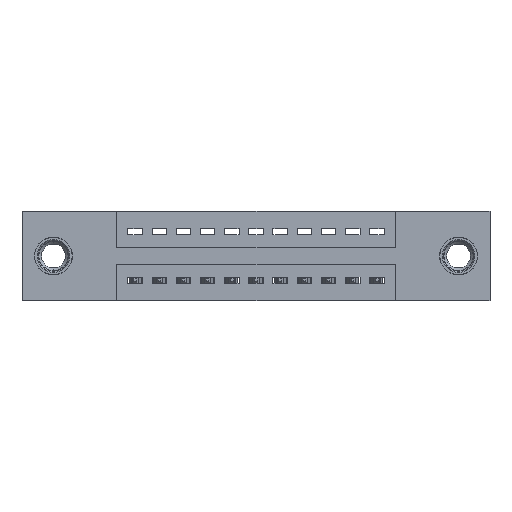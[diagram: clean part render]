
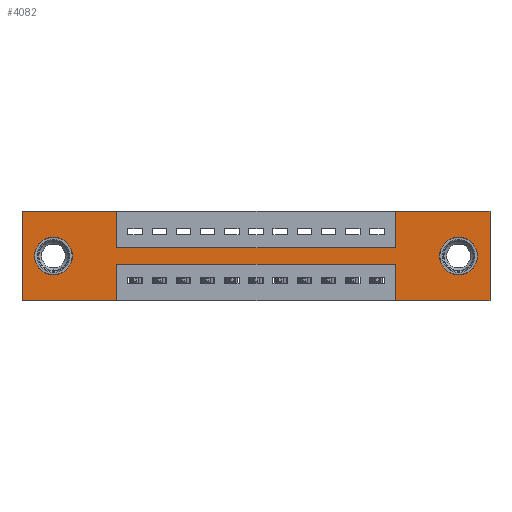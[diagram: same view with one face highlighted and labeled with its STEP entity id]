
A CAD part, front view. The second image highlights one B-rep face of the part: STEP entity #4082.
In plain terms, the highlighted planar face has unit normal (0, -1, 0).
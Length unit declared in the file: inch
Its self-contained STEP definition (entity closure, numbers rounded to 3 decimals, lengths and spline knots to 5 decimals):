
#13 = CARTESIAN_POINT ( 'NONE',  ( 0.3925, 0., -0.22 ) ) ;
#26 = CARTESIAN_POINT ( 'NONE',  ( 0.3925, 0., 0. ) ) ;
#40 = EDGE_CURVE ( 'NONE', #13042, #10069, #11287, .T. ) ;
#280 = ORIENTED_EDGE ( 'NONE', *, *, #3302, .F. ) ;
#438 = DIRECTION ( 'NONE',  ( 0., 0., 1. ) ) ;
#495 = CARTESIAN_POINT ( 'NONE',  ( 0.13, 0., -0.185 ) ) ;
#990 = VERTEX_POINT ( 'NONE', #8089 ) ;
#1061 = CARTESIAN_POINT ( 'NONE',  ( 1.805, 0., -0.185 ) ) ;
#1088 = LINE ( 'NONE', #1348, #12640 ) ;
#1348 = CARTESIAN_POINT ( 'NONE',  ( 0., 0., 0. ) ) ;
#1362 = LINE ( 'NONE', #9178, #10971 ) ;
#1451 = CARTESIAN_POINT ( 'NONE',  ( 0., 0., 0. ) ) ;
#1466 = LINE ( 'NONE', #7361, #10220 ) ;
#1479 = CARTESIAN_POINT ( 'NONE',  ( 0.3925, 0., -0.22 ) ) ;
#1532 = VERTEX_POINT ( 'NONE', #8719 ) ;
#1937 = LINE ( 'NONE', #2942, #3266 ) ;
#1959 = CARTESIAN_POINT ( 'NONE',  ( 1.5425, 0., -0.37 ) ) ;
#2083 = CARTESIAN_POINT ( 'NONE',  ( 1.805, 0., -0.263 ) ) ;
#2145 = DIRECTION ( 'NONE',  ( 0., -1., 0. ) ) ;
#2225 = EDGE_CURVE ( 'NONE', #10069, #12601, #1362, .T. ) ;
#2323 = EDGE_CURVE ( 'NONE', #13293, #8570, #8824, .T. ) ;
#2640 = EDGE_CURVE ( 'NONE', #3064, #1532, #7993, .T. ) ;
#2713 = VERTEX_POINT ( 'NONE', #13550 ) ;
#2833 = DIRECTION ( 'NONE',  ( 0., 0., 1. ) ) ;
#2881 = VECTOR ( 'NONE', #11647, 39.37008 ) ;
#2925 = CIRCLE ( 'NONE', #8544, 0.078 ) ;
#2942 = CARTESIAN_POINT ( 'NONE',  ( 1.935, 0., 0. ) ) ;
#3064 = VERTEX_POINT ( 'NONE', #8802 ) ;
#3232 = DIRECTION ( 'NONE',  ( 0., 0., -1. ) ) ;
#3266 = VECTOR ( 'NONE', #9234, 39.37008 ) ;
#3302 = EDGE_CURVE ( 'NONE', #8677, #11229, #7288, .T. ) ;
#3364 = EDGE_LOOP ( 'NONE', ( #7395, #4748 ) ) ;
#3522 = LINE ( 'NONE', #13420, #6992 ) ;
#3892 = DIRECTION ( 'NONE',  ( 1., 0., 0. ) ) ;
#3948 = FACE_BOUND ( 'NONE', #3364, .T. ) ;
#3956 = DIRECTION ( 'NONE',  ( 0., 0., 1. ) ) ;
#4082 = ADVANCED_FACE ( 'NONE', ( #8427, #3948, #11879 ), #10182, .T. ) ;
#4088 = CARTESIAN_POINT ( 'NONE',  ( 1.805, 0., -0.107 ) ) ;
#4175 = EDGE_CURVE ( 'NONE', #9223, #8423, #6757, .T. ) ;
#4223 = CARTESIAN_POINT ( 'NONE',  ( 0., 0., -0.37 ) ) ;
#4258 = DIRECTION ( 'NONE',  ( 0., 1., 0. ) ) ;
#4269 = DIRECTION ( 'NONE',  ( 0., 0., 1. ) ) ;
#4323 = VECTOR ( 'NONE', #3956, 39.37008 ) ;
#4337 = ORIENTED_EDGE ( 'NONE', *, *, #7626, .F. ) ;
#4462 = VECTOR ( 'NONE', #8029, 39.37008 ) ;
#4523 = EDGE_CURVE ( 'NONE', #7480, #12396, #13524, .T. ) ;
#4541 = EDGE_CURVE ( 'NONE', #9490, #8677, #1466, .T. ) ;
#4584 = ORIENTED_EDGE ( 'NONE', *, *, #40, .F. ) ;
#4748 = ORIENTED_EDGE ( 'NONE', *, *, #2640, .T. ) ;
#5036 = VECTOR ( 'NONE', #7605, 39.37008 ) ;
#5208 = ORIENTED_EDGE ( 'NONE', *, *, #4175, .F. ) ;
#5555 = CIRCLE ( 'NONE', #7298, 0.078 ) ;
#5570 = EDGE_LOOP ( 'NONE', ( #5208, #8918, #280, #5935, #10396, #7693, #4584, #12400, #11058, #8085, #10325, #4337 ) ) ;
#5607 = EDGE_CURVE ( 'NONE', #12396, #7480, #2925, .T. ) ;
#5935 = ORIENTED_EDGE ( 'NONE', *, *, #4541, .F. ) ;
#5956 = AXIS2_PLACEMENT_3D ( 'NONE', #4223, #2145, #9364 ) ;
#6016 = LINE ( 'NONE', #12966, #5036 ) ;
#6119 = DIRECTION ( 'NONE',  ( 0., 0., 1. ) ) ;
#6484 = VECTOR ( 'NONE', #12430, 39.37008 ) ;
#6572 = CARTESIAN_POINT ( 'NONE',  ( 1.5425, 0., -0.22 ) ) ;
#6757 = LINE ( 'NONE', #12187, #4462 ) ;
#6992 = VECTOR ( 'NONE', #8454, 39.37008 ) ;
#7288 = LINE ( 'NONE', #1959, #12718 ) ;
#7298 = AXIS2_PLACEMENT_3D ( 'NONE', #12323, #9262, #2833 ) ;
#7361 = CARTESIAN_POINT ( 'NONE',  ( 0., 0., -0.37 ) ) ;
#7395 = ORIENTED_EDGE ( 'NONE', *, *, #12686, .T. ) ;
#7463 = EDGE_CURVE ( 'NONE', #11229, #9223, #8041, .T. ) ;
#7480 = VERTEX_POINT ( 'NONE', #2083 ) ;
#7605 = DIRECTION ( 'NONE',  ( -1., 0., 0. ) ) ;
#7626 = EDGE_CURVE ( 'NONE', #8423, #2713, #6016, .T. ) ;
#7693 = ORIENTED_EDGE ( 'NONE', *, *, #2225, .F. ) ;
#7947 = EDGE_CURVE ( 'NONE', #8570, #13042, #3522, .T. ) ;
#7993 = CIRCLE ( 'NONE', #8354, 0.078 ) ;
#8029 = DIRECTION ( 'NONE',  ( 0., 0., -1. ) ) ;
#8041 = LINE ( 'NONE', #13, #2881 ) ;
#8085 = ORIENTED_EDGE ( 'NONE', *, *, #12481, .F. ) ;
#8089 = CARTESIAN_POINT ( 'NONE',  ( 0., 0., 0. ) ) ;
#8224 = CARTESIAN_POINT ( 'NONE',  ( 0.3925, 0., 0. ) ) ;
#8294 = DIRECTION ( 'NONE',  ( 0., 1., 0. ) ) ;
#8354 = AXIS2_PLACEMENT_3D ( 'NONE', #495, #13401, #4269 ) ;
#8421 = CARTESIAN_POINT ( 'NONE',  ( 1.5425, 0., 0. ) ) ;
#8423 = VERTEX_POINT ( 'NONE', #13218 ) ;
#8427 = FACE_BOUND ( 'NONE', #9754, .T. ) ;
#8454 = DIRECTION ( 'NONE',  ( 1., 0., 0. ) ) ;
#8544 = AXIS2_PLACEMENT_3D ( 'NONE', #10350, #8294, #12407 ) ;
#8559 = CARTESIAN_POINT ( 'NONE',  ( 1.5425, 0., -0.37 ) ) ;
#8570 = VERTEX_POINT ( 'NONE', #10160 ) ;
#8658 = CARTESIAN_POINT ( 'NONE',  ( 1.935, 0., -0.37 ) ) ;
#8677 = VERTEX_POINT ( 'NONE', #8559 ) ;
#8719 = CARTESIAN_POINT ( 'NONE',  ( 0.13, 0., -0.107 ) ) ;
#8802 = CARTESIAN_POINT ( 'NONE',  ( 0.13, 0., -0.263 ) ) ;
#8824 = LINE ( 'NONE', #8224, #6484 ) ;
#8918 = ORIENTED_EDGE ( 'NONE', *, *, #7463, .F. ) ;
#8929 = CARTESIAN_POINT ( 'NONE',  ( 1.5425, 0., -0.15 ) ) ;
#9178 = CARTESIAN_POINT ( 'NONE',  ( 0., 0., 0. ) ) ;
#9223 = VERTEX_POINT ( 'NONE', #1479 ) ;
#9234 = DIRECTION ( 'NONE',  ( 0., 0., -1. ) ) ;
#9262 = DIRECTION ( 'NONE',  ( 0., 1., 0. ) ) ;
#9364 = DIRECTION ( 'NONE',  ( 0., 0., -1. ) ) ;
#9477 = DIRECTION ( 'NONE',  ( -1., 0., 0. ) ) ;
#9490 = VERTEX_POINT ( 'NONE', #8658 ) ;
#9580 = AXIS2_PLACEMENT_3D ( 'NONE', #1061, #4258, #3232 ) ;
#9668 = DIRECTION ( 'NONE',  ( 1., 0., 0. ) ) ;
#9754 = EDGE_LOOP ( 'NONE', ( #10500, #10192 ) ) ;
#10069 = VERTEX_POINT ( 'NONE', #8421 ) ;
#10160 = CARTESIAN_POINT ( 'NONE',  ( 0.3925, 0., -0.15 ) ) ;
#10182 = PLANE ( 'NONE',  #5956 ) ;
#10192 = ORIENTED_EDGE ( 'NONE', *, *, #4523, .T. ) ;
#10220 = VECTOR ( 'NONE', #9477, 39.37008 ) ;
#10325 = ORIENTED_EDGE ( 'NONE', *, *, #13562, .F. ) ;
#10350 = CARTESIAN_POINT ( 'NONE',  ( 1.805, 0., -0.185 ) ) ;
#10396 = ORIENTED_EDGE ( 'NONE', *, *, #11669, .F. ) ;
#10500 = ORIENTED_EDGE ( 'NONE', *, *, #5607, .T. ) ;
#10971 = VECTOR ( 'NONE', #3892, 39.37008 ) ;
#11058 = ORIENTED_EDGE ( 'NONE', *, *, #2323, .F. ) ;
#11229 = VERTEX_POINT ( 'NONE', #6572 ) ;
#11287 = LINE ( 'NONE', #13555, #4323 ) ;
#11647 = DIRECTION ( 'NONE',  ( -1., 0., 0. ) ) ;
#11669 = EDGE_CURVE ( 'NONE', #12601, #9490, #1937, .T. ) ;
#11879 = FACE_OUTER_BOUND ( 'NONE', #5570, .T. ) ;
#12145 = CARTESIAN_POINT ( 'NONE',  ( 1.935, 0., 0. ) ) ;
#12187 = CARTESIAN_POINT ( 'NONE',  ( 0.3925, 0., -0.37 ) ) ;
#12323 = CARTESIAN_POINT ( 'NONE',  ( 0.13, 0., -0.185 ) ) ;
#12396 = VERTEX_POINT ( 'NONE', #4088 ) ;
#12400 = ORIENTED_EDGE ( 'NONE', *, *, #7947, .F. ) ;
#12407 = DIRECTION ( 'NONE',  ( 0., 0., -1. ) ) ;
#12430 = DIRECTION ( 'NONE',  ( 0., 0., -1. ) ) ;
#12481 = EDGE_CURVE ( 'NONE', #990, #13293, #1088, .T. ) ;
#12601 = VERTEX_POINT ( 'NONE', #12145 ) ;
#12640 = VECTOR ( 'NONE', #9668, 39.37008 ) ;
#12686 = EDGE_CURVE ( 'NONE', #1532, #3064, #5555, .T. ) ;
#12718 = VECTOR ( 'NONE', #6119, 39.37008 ) ;
#12966 = CARTESIAN_POINT ( 'NONE',  ( 0., 0., -0.37 ) ) ;
#13042 = VERTEX_POINT ( 'NONE', #8929 ) ;
#13218 = CARTESIAN_POINT ( 'NONE',  ( 0.3925, 0., -0.37 ) ) ;
#13293 = VERTEX_POINT ( 'NONE', #26 ) ;
#13302 = LINE ( 'NONE', #1451, #13465 ) ;
#13401 = DIRECTION ( 'NONE',  ( 0., 1., 0. ) ) ;
#13420 = CARTESIAN_POINT ( 'NONE',  ( 0.3925, 0., -0.15 ) ) ;
#13465 = VECTOR ( 'NONE', #438, 39.37008 ) ;
#13524 = CIRCLE ( 'NONE', #9580, 0.078 ) ;
#13550 = CARTESIAN_POINT ( 'NONE',  ( 0., 0., -0.37 ) ) ;
#13555 = CARTESIAN_POINT ( 'NONE',  ( 1.5425, 0., 0. ) ) ;
#13562 = EDGE_CURVE ( 'NONE', #2713, #990, #13302, .T. ) ;
